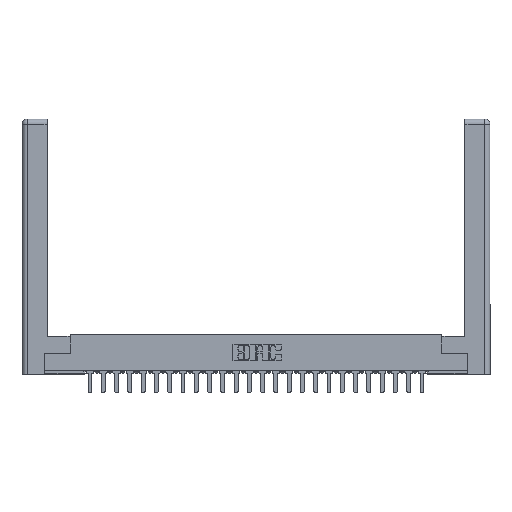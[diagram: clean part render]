
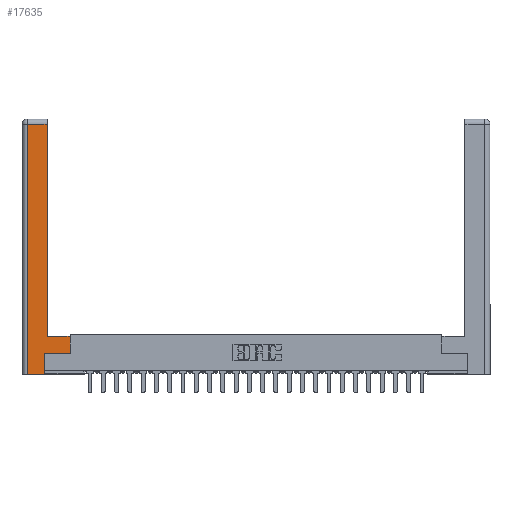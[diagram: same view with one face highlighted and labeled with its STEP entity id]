
A CAD part, top view. The second image highlights one B-rep face of the part: STEP entity #17635.
In plain terms, the highlighted planar face has unit normal (0, 0, 1).
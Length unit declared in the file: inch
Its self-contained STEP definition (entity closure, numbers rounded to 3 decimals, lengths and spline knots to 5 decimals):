
#1420 = AXIS2_PLACEMENT_3D ( 'NONE', #3432, #9541, #22332 ) ;
#2054 = CARTESIAN_POINT ( 'NONE',  ( 0.265, 0., 0. ) ) ;
#2118 = CARTESIAN_POINT ( 'NONE',  ( 0.565, 0.45, 0. ) ) ;
#2455 = VECTOR ( 'NONE', #11863, 39.37008 ) ;
#2845 = DIRECTION ( 'NONE',  ( 0., 1., 0. ) ) ;
#3337 = VECTOR ( 'NONE', #2845, 39.37008 ) ;
#3432 = CARTESIAN_POINT ( 'NONE',  ( 0., 0., 0. ) ) ;
#4162 = VECTOR ( 'NONE', #19977, 39.37008 ) ;
#4560 = VERTEX_POINT ( 'NONE', #20037 ) ;
#5109 = FACE_OUTER_BOUND ( 'NONE', #16403, .T. ) ;
#5914 = EDGE_CURVE ( 'NONE', #17864, #27474, #26284, .T. ) ;
#6715 = LINE ( 'NONE', #11643, #3337 ) ;
#7225 = CARTESIAN_POINT ( 'NONE',  ( 0.265, 0., 0. ) ) ;
#7571 = ORIENTED_EDGE ( 'NONE', *, *, #14438, .T. ) ;
#8439 = VERTEX_POINT ( 'NONE', #17545 ) ;
#8835 = LINE ( 'NONE', #12129, #2455 ) ;
#8966 = CARTESIAN_POINT ( 'NONE',  ( 0.265, 0.245, 0. ) ) ;
#9254 = DIRECTION ( 'NONE',  ( -1., 0., 0. ) ) ;
#9347 = PLANE ( 'NONE',  #1420 ) ;
#9541 = DIRECTION ( 'NONE',  ( 0., 0., -1. ) ) ;
#9855 = ORIENTED_EDGE ( 'NONE', *, *, #24567, .T. ) ;
#9976 = LINE ( 'NONE', #14854, #27691 ) ;
#10252 = CARTESIAN_POINT ( 'NONE',  ( 0.0615, 0., 0. ) ) ;
#10350 = ORIENTED_EDGE ( 'NONE', *, *, #22444, .T. ) ;
#10637 = LINE ( 'NONE', #13885, #12967 ) ;
#10781 = ORIENTED_EDGE ( 'NONE', *, *, #11471, .T. ) ;
#10900 = LINE ( 'NONE', #23521, #21918 ) ;
#11243 = ORIENTED_EDGE ( 'NONE', *, *, #26373, .T. ) ;
#11284 = CARTESIAN_POINT ( 'NONE',  ( 0.565, 0.245, 0. ) ) ;
#11471 = EDGE_CURVE ( 'NONE', #25307, #18030, #8835, .T. ) ;
#11643 = CARTESIAN_POINT ( 'NONE',  ( 0.295, 3., 0. ) ) ;
#11863 = DIRECTION ( 'NONE',  ( 0., 1., 0. ) ) ;
#11970 = EDGE_CURVE ( 'NONE', #18030, #8439, #21235, .T. ) ;
#12129 = CARTESIAN_POINT ( 'NONE',  ( 0.265, 0.245, 0. ) ) ;
#12296 = CARTESIAN_POINT ( 'NONE',  ( 0.295, 0.45, 0. ) ) ;
#12680 = DIRECTION ( 'NONE',  ( 0., -1., 0. ) ) ;
#12967 = VECTOR ( 'NONE', #16041, 39.37008 ) ;
#13366 = DIRECTION ( 'NONE',  ( -1., 0., 0. ) ) ;
#13885 = CARTESIAN_POINT ( 'NONE',  ( 0.565, 0.45, 0. ) ) ;
#13998 = CARTESIAN_POINT ( 'NONE',  ( 0.0615, 2.94, 0. ) ) ;
#14438 = EDGE_CURVE ( 'NONE', #27474, #4560, #6715, .T. ) ;
#14854 = CARTESIAN_POINT ( 'NONE',  ( 0.0615, 0., 0. ) ) ;
#15106 = EDGE_CURVE ( 'NONE', #8439, #17864, #10637, .T. ) ;
#15166 = LINE ( 'NONE', #2054, #20156 ) ;
#15875 = VERTEX_POINT ( 'NONE', #10252 ) ;
#15939 = VECTOR ( 'NONE', #9254, 39.37008 ) ;
#16041 = DIRECTION ( 'NONE',  ( 0., 1., 0. ) ) ;
#16403 = EDGE_LOOP ( 'NONE', ( #7571, #9855, #10350, #11243, #10781, #22653, #23254, #18651 ) ) ;
#17545 = CARTESIAN_POINT ( 'NONE',  ( 0.565, 0.245, 0. ) ) ;
#17635 = ADVANCED_FACE ( 'NONE', ( #5109 ), #9347, .F. ) ;
#17864 = VERTEX_POINT ( 'NONE', #2118 ) ;
#18030 = VERTEX_POINT ( 'NONE', #8966 ) ;
#18651 = ORIENTED_EDGE ( 'NONE', *, *, #5914, .T. ) ;
#18867 = DIRECTION ( 'NONE',  ( 1., 0., 0. ) ) ;
#18914 = VERTEX_POINT ( 'NONE', #13998 ) ;
#19977 = DIRECTION ( 'NONE',  ( 1., 0., 0. ) ) ;
#20037 = CARTESIAN_POINT ( 'NONE',  ( 0.295, 2.94, 0. ) ) ;
#20156 = VECTOR ( 'NONE', #18867, 39.37008 ) ;
#21235 = LINE ( 'NONE', #11284, #4162 ) ;
#21918 = VECTOR ( 'NONE', #13366, 39.37008 ) ;
#22332 = DIRECTION ( 'NONE',  ( -1., 0., 0. ) ) ;
#22444 = EDGE_CURVE ( 'NONE', #18914, #15875, #9976, .T. ) ;
#22653 = ORIENTED_EDGE ( 'NONE', *, *, #11970, .T. ) ;
#23254 = ORIENTED_EDGE ( 'NONE', *, *, #15106, .T. ) ;
#23521 = CARTESIAN_POINT ( 'NONE',  ( 0.0615, 2.94, 0. ) ) ;
#24567 = EDGE_CURVE ( 'NONE', #4560, #18914, #10900, .T. ) ;
#25307 = VERTEX_POINT ( 'NONE', #7225 ) ;
#26173 = CARTESIAN_POINT ( 'NONE',  ( 0.295, 0.45, 0. ) ) ;
#26284 = LINE ( 'NONE', #26173, #15939 ) ;
#26373 = EDGE_CURVE ( 'NONE', #15875, #25307, #15166, .T. ) ;
#27474 = VERTEX_POINT ( 'NONE', #12296 ) ;
#27691 = VECTOR ( 'NONE', #12680, 39.37008 ) ;
